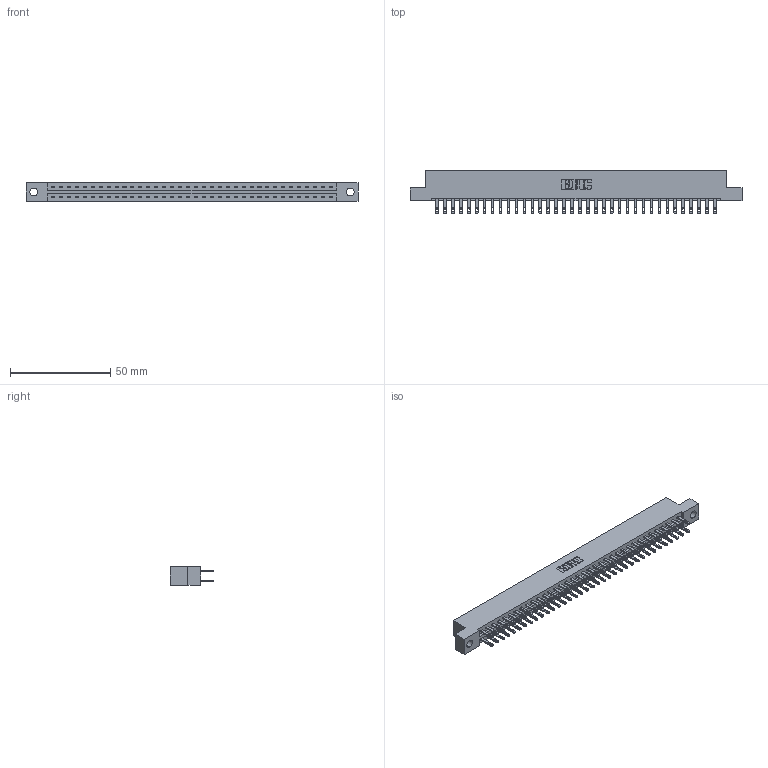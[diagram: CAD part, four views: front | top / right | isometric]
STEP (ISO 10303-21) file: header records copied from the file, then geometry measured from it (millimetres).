
FILE_DESCRIPTION (( 'STEP AP203' ), '1' );
FILE_NAME ('887-072-500-204.STEP', '2020-09-21T03:24:20', ( '' ), ( '' ), 'SwSTEP 2.0', 'SolidWorks 2020', '' );
FILE_SCHEMA (( 'CONFIG_CONTROL_DESIGN' ));
Length unit declared in the file: inch
Products named in the file (3): 837 Part_Flush Mounting Lugs - 0.156 Dia-TH; 345-292-001_345-293-100; 887-072-500-204
Assembly tree (73 placements, depth 2):
  887-072-500-204
    837 Part_Flush Mounting Lugs - 0.156 Dia-TH
    345-292-001_345-293-100  x72
Bounding box: 165.66 x 21.85 x 9.4 mm (x, y, z)
Volume: 17510.7 mm3; surface area: 20333.9 mm2
Topology: 73 solids, 73 shells, 3714 faces, 11327 edges, 7550 vertices
Faces by surface type: plane 2374, cylinder 1340
Entity records: 28621 total; most frequent: CARTESIAN_POINT 4826, ORIENTED_EDGE 4762, DIRECTION 4117, EDGE_CURVE 2381, VECTOR 2249, LINE 2249, VERTEX_POINT 1586, AXIS2_PLACEMENT_3D 934
